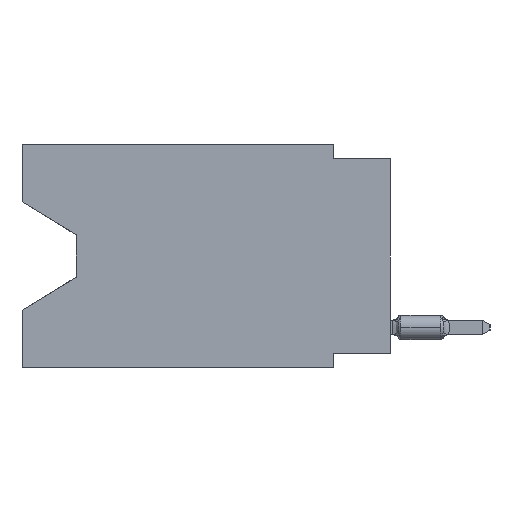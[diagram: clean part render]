
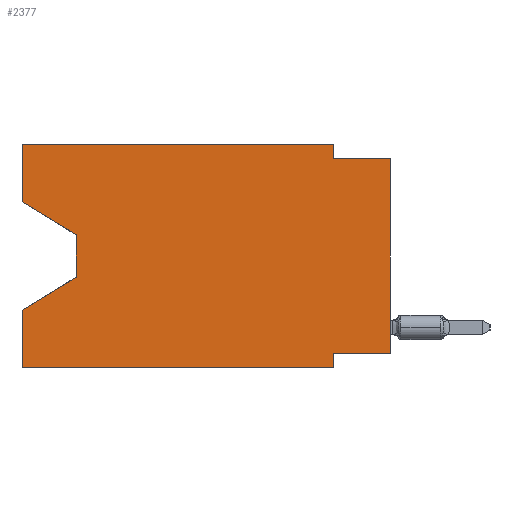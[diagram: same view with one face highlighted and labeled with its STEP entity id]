
A CAD part, left-side view. The second image highlights one B-rep face of the part: STEP entity #2377.
In plain terms, the highlighted planar face has unit normal (-1, 0, 0).
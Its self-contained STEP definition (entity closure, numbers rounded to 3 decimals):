
#2377 = ADVANCED_FACE ( 'NONE', ( #9303 ), #3759, .F. ) ;
#3759 = PLANE ( 'NONE',  #62455 ) ;
#5849 = CARTESIAN_POINT ( 'NONE',  ( 0., 16.383, 0. ) ) ;
#6561 = EDGE_CURVE ( 'NONE', #42272, #50038, #50747, .T. ) ;
#6866 = CARTESIAN_POINT ( 'NONE',  ( 0., 13.97, -5.893 ) ) ;
#6923 = LINE ( 'NONE', #36101, #46963 ) ;
#8376 = EDGE_CURVE ( 'NONE', #32493, #17219, #53282, .T. ) ;
#8581 = DIRECTION ( 'NONE',  ( 0., -1., 0. ) ) ;
#8679 = ORIENTED_EDGE ( 'NONE', *, *, #8376, .T. ) ;
#8956 = LINE ( 'NONE', #42914, #70162 ) ;
#9303 = FACE_OUTER_BOUND ( 'NONE', #31040, .T. ) ;
#9597 = CARTESIAN_POINT ( 'NONE',  ( 0., 0., 0. ) ) ;
#9664 = EDGE_CURVE ( 'NONE', #50038, #17219, #8956, .T. ) ;
#9777 = CARTESIAN_POINT ( 'NONE',  ( 0., 16.383, -2.546 ) ) ;
#10375 = EDGE_CURVE ( 'NONE', #66779, #59969, #32305, .T. ) ;
#14112 = CARTESIAN_POINT ( 'NONE',  ( 0., 16.383, -7.36 ) ) ;
#14230 = LINE ( 'NONE', #36384, #40987 ) ;
#15213 = CARTESIAN_POINT ( 'NONE',  ( 0., 16.383, -9.906 ) ) ;
#17159 = VECTOR ( 'NONE', #35139, 1000. ) ;
#17219 = VERTEX_POINT ( 'NONE', #68204 ) ;
#17541 = ORIENTED_EDGE ( 'NONE', *, *, #6561, .F. ) ;
#18139 = CARTESIAN_POINT ( 'NONE',  ( 0., 16.383, 0. ) ) ;
#18541 = VERTEX_POINT ( 'NONE', #34146 ) ;
#19762 = DIRECTION ( 'NONE',  ( 0., -1., 0. ) ) ;
#20170 = VECTOR ( 'NONE', #27645, 1000. ) ;
#20377 = VECTOR ( 'NONE', #35224, 1000. ) ;
#21405 = EDGE_CURVE ( 'NONE', #66779, #66915, #6923, .T. ) ;
#22807 = ORIENTED_EDGE ( 'NONE', *, *, #39122, .F. ) ;
#23031 = DIRECTION ( 'NONE',  ( 0., 1., 0. ) ) ;
#23806 = CARTESIAN_POINT ( 'NONE',  ( 0., 2.54, 0. ) ) ;
#23951 = CARTESIAN_POINT ( 'NONE',  ( 0., 13.97, -5.893 ) ) ;
#24512 = ORIENTED_EDGE ( 'NONE', *, *, #50498, .F. ) ;
#25153 = EDGE_CURVE ( 'NONE', #59969, #67420, #67522, .T. ) ;
#26196 = CARTESIAN_POINT ( 'NONE',  ( 0., 16.383, -2.546 ) ) ;
#26246 = EDGE_CURVE ( 'NONE', #42272, #18541, #49453, .T. ) ;
#27107 = VERTEX_POINT ( 'NONE', #14112 ) ;
#27645 = DIRECTION ( 'NONE',  ( 0., 0., -1. ) ) ;
#29223 = LINE ( 'NONE', #18139, #17159 ) ;
#31040 = EDGE_LOOP ( 'NONE', ( #46245, #65691, #40762, #24512, #8679, #48865, #17541, #46573, #22807, #55223, #47270, #56704 ) ) ;
#31093 = VECTOR ( 'NONE', #72005, 1000. ) ;
#32305 = LINE ( 'NONE', #9777, #33791 ) ;
#32399 = VECTOR ( 'NONE', #69244, 1000. ) ;
#32493 = VERTEX_POINT ( 'NONE', #15213 ) ;
#33791 = VECTOR ( 'NONE', #60014, 1000. ) ;
#34146 = CARTESIAN_POINT ( 'NONE',  ( 0., 0., -0.635 ) ) ;
#34491 = CARTESIAN_POINT ( 'NONE',  ( 0., 0., -0.635 ) ) ;
#35139 = DIRECTION ( 'NONE',  ( 0., 0., 1. ) ) ;
#35224 = DIRECTION ( 'NONE',  ( 0., -1., 0. ) ) ;
#36101 = CARTESIAN_POINT ( 'NONE',  ( 0., 16.383, 0. ) ) ;
#36384 = CARTESIAN_POINT ( 'NONE',  ( 0., 16.383, 0. ) ) ;
#36454 = DIRECTION ( 'NONE',  ( 0., 0., 1. ) ) ;
#39122 = EDGE_CURVE ( 'NONE', #46668, #18541, #68836, .T. ) ;
#39541 = EDGE_CURVE ( 'NONE', #67420, #27107, #63110, .T. ) ;
#39663 = CARTESIAN_POINT ( 'NONE',  ( 0., 2.54, -9.271 ) ) ;
#40580 = DIRECTION ( 'NONE',  ( 0., 0.855, -0.519 ) ) ;
#40762 = ORIENTED_EDGE ( 'NONE', *, *, #39541, .T. ) ;
#40987 = VECTOR ( 'NONE', #19762, 1000. ) ;
#41685 = VECTOR ( 'NONE', #40580, 1000. ) ;
#41825 = DIRECTION ( 'NONE',  ( 1., 0., 0. ) ) ;
#42272 = VERTEX_POINT ( 'NONE', #54329 ) ;
#42914 = CARTESIAN_POINT ( 'NONE',  ( 0., 2.54, -9.906 ) ) ;
#44042 = VECTOR ( 'NONE', #8581, 1000. ) ;
#45224 = LINE ( 'NONE', #23806, #32399 ) ;
#46245 = ORIENTED_EDGE ( 'NONE', *, *, #10375, .T. ) ;
#46573 = ORIENTED_EDGE ( 'NONE', *, *, #26246, .T. ) ;
#46668 = VERTEX_POINT ( 'NONE', #59671 ) ;
#46963 = VECTOR ( 'NONE', #36454, 1000. ) ;
#47270 = ORIENTED_EDGE ( 'NONE', *, *, #54688, .F. ) ;
#48447 = CARTESIAN_POINT ( 'NONE',  ( 0., 16.383, -9.906 ) ) ;
#48865 = ORIENTED_EDGE ( 'NONE', *, *, #9664, .F. ) ;
#49453 = LINE ( 'NONE', #9597, #31093 ) ;
#50038 = VERTEX_POINT ( 'NONE', #39663 ) ;
#50498 = EDGE_CURVE ( 'NONE', #32493, #27107, #29223, .T. ) ;
#50747 = LINE ( 'NONE', #61831, #65243 ) ;
#50968 = EDGE_CURVE ( 'NONE', #52457, #46668, #45224, .T. ) ;
#52457 = VERTEX_POINT ( 'NONE', #65598 ) ;
#53282 = LINE ( 'NONE', #48447, #44042 ) ;
#54329 = CARTESIAN_POINT ( 'NONE',  ( 0., 0., -9.271 ) ) ;
#54369 = CARTESIAN_POINT ( 'NONE',  ( 0., 16.383, 0. ) ) ;
#54688 = EDGE_CURVE ( 'NONE', #66915, #52457, #14230, .T. ) ;
#55223 = ORIENTED_EDGE ( 'NONE', *, *, #50968, .F. ) ;
#56704 = ORIENTED_EDGE ( 'NONE', *, *, #21405, .F. ) ;
#59671 = CARTESIAN_POINT ( 'NONE',  ( 0., 2.54, -0.635 ) ) ;
#59969 = VERTEX_POINT ( 'NONE', #70234 ) ;
#60014 = DIRECTION ( 'NONE',  ( 0., -0.855, -0.519 ) ) ;
#61831 = CARTESIAN_POINT ( 'NONE',  ( 0., 0., -9.271 ) ) ;
#62340 = CARTESIAN_POINT ( 'NONE',  ( 0., 13.97, -4.013 ) ) ;
#62455 = AXIS2_PLACEMENT_3D ( 'NONE', #54369, #41825, #70627 ) ;
#63110 = LINE ( 'NONE', #23951, #41685 ) ;
#65243 = VECTOR ( 'NONE', #23031, 1000. ) ;
#65443 = DIRECTION ( 'NONE',  ( 0., 0., -1. ) ) ;
#65598 = CARTESIAN_POINT ( 'NONE',  ( 0., 2.54, 0. ) ) ;
#65691 = ORIENTED_EDGE ( 'NONE', *, *, #25153, .T. ) ;
#66779 = VERTEX_POINT ( 'NONE', #26196 ) ;
#66915 = VERTEX_POINT ( 'NONE', #5849 ) ;
#67420 = VERTEX_POINT ( 'NONE', #6866 ) ;
#67522 = LINE ( 'NONE', #62340, #20170 ) ;
#68204 = CARTESIAN_POINT ( 'NONE',  ( 0., 2.54, -9.906 ) ) ;
#68836 = LINE ( 'NONE', #34491, #20377 ) ;
#69244 = DIRECTION ( 'NONE',  ( 0., 0., -1. ) ) ;
#70162 = VECTOR ( 'NONE', #65443, 1000. ) ;
#70234 = CARTESIAN_POINT ( 'NONE',  ( 0., 13.97, -4.013 ) ) ;
#70627 = DIRECTION ( 'NONE',  ( 0., 0., -1. ) ) ;
#72005 = DIRECTION ( 'NONE',  ( 0., 0., 1. ) ) ;
